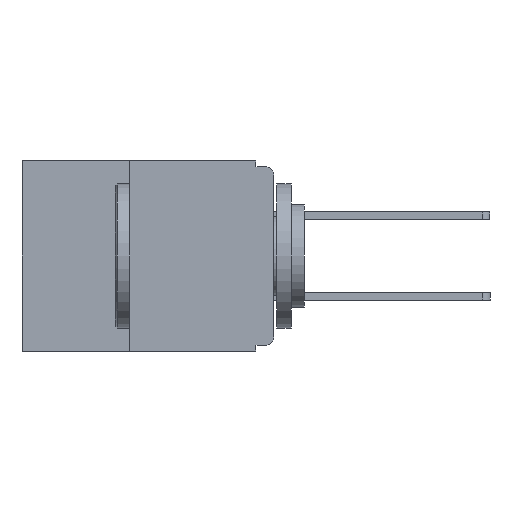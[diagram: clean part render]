
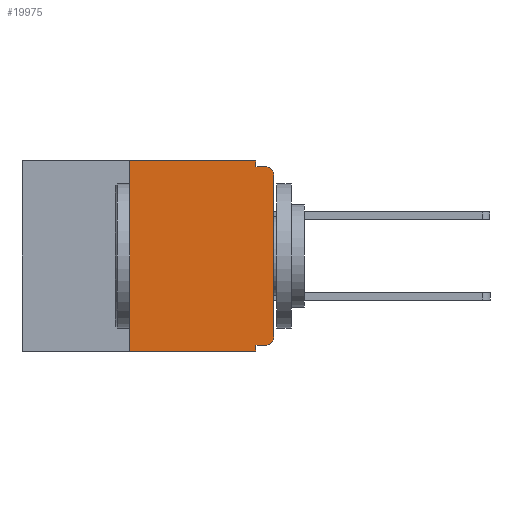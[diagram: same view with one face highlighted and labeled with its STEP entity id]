
A CAD part, left-side view. The second image highlights one B-rep face of the part: STEP entity #19975.
In plain terms, the highlighted planar face has unit normal (-1, 0, 0).
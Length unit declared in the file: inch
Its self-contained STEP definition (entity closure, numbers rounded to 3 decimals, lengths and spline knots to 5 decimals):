
#14 = DIRECTION ( 'NONE',  ( 0., 0., 1. ) ) ;
#319 = PLANE ( 'NONE',  #8817 ) ;
#542 = VERTEX_POINT ( 'NONE', #6437 ) ;
#601 = EDGE_CURVE ( 'NONE', #12210, #19480, #27100, .T. ) ;
#2142 = CARTESIAN_POINT ( 'NONE',  ( 0., 0.25, -0.33 ) ) ;
#2256 = EDGE_CURVE ( 'NONE', #4718, #12210, #6326, .T. ) ;
#2502 = LINE ( 'NONE', #9991, #25057 ) ;
#2590 = CARTESIAN_POINT ( 'NONE',  ( 0., 0.437, 0. ) ) ;
#2668 = DIRECTION ( 'NONE',  ( 0., -1., 0. ) ) ;
#2788 = CARTESIAN_POINT ( 'NONE',  ( 0., 0.25, -0.33 ) ) ;
#2958 = EDGE_LOOP ( 'NONE', ( #22342, #22671, #18648, #22723, #16633, #20723, #24435, #16682, #3962, #11297 ) ) ;
#2968 = VERTEX_POINT ( 'NONE', #4401 ) ;
#3151 = CARTESIAN_POINT ( 'NONE',  ( 0., 0., -0.32 ) ) ;
#3210 = CARTESIAN_POINT ( 'NONE',  ( 0., 0.031, -0.33 ) ) ;
#3430 = DIRECTION ( 'NONE',  ( 0., 0., -1. ) ) ;
#3502 = DIRECTION ( 'NONE',  ( 0., -1., 0. ) ) ;
#3962 = ORIENTED_EDGE ( 'NONE', *, *, #23282, .F. ) ;
#4376 = DIRECTION ( 'NONE',  ( 0., 0., 1. ) ) ;
#4401 = CARTESIAN_POINT ( 'NONE',  ( 0., 0.031, -0.32 ) ) ;
#4718 = VERTEX_POINT ( 'NONE', #13551 ) ;
#4810 = DIRECTION ( 'NONE',  ( 1., 0., 0. ) ) ;
#4890 = CARTESIAN_POINT ( 'NONE',  ( 0., 0.437, -0.33 ) ) ;
#5719 = VERTEX_POINT ( 'NONE', #17466 ) ;
#6326 = LINE ( 'NONE', #17596, #15929 ) ;
#6437 = CARTESIAN_POINT ( 'NONE',  ( 0., 0., -0.025 ) ) ;
#6845 = VECTOR ( 'NONE', #25123, 39.37008 ) ;
#7030 = DIRECTION ( 'NONE',  ( -1., 0., 0. ) ) ;
#7438 = CIRCLE ( 'NONE', #10434, 0.015 ) ;
#7445 = VECTOR ( 'NONE', #4376, 39.37008 ) ;
#8817 = AXIS2_PLACEMENT_3D ( 'NONE', #2590, #4810, #20133 ) ;
#8823 = VECTOR ( 'NONE', #2668, 39.37008 ) ;
#9991 = CARTESIAN_POINT ( 'NONE',  ( 0., 0.031, -0.33 ) ) ;
#10374 = CIRCLE ( 'NONE', #20193, 0.015 ) ;
#10434 = AXIS2_PLACEMENT_3D ( 'NONE', #11715, #26837, #13908 ) ;
#10545 = EDGE_CURVE ( 'NONE', #2968, #20801, #2502, .T. ) ;
#11297 = ORIENTED_EDGE ( 'NONE', *, *, #11732, .T. ) ;
#11715 = CARTESIAN_POINT ( 'NONE',  ( 0., 0.015, -0.025 ) ) ;
#11732 = EDGE_CURVE ( 'NONE', #14451, #21598, #10374, .T. ) ;
#12210 = VERTEX_POINT ( 'NONE', #15131 ) ;
#12665 = LINE ( 'NONE', #16422, #6845 ) ;
#13256 = LINE ( 'NONE', #2142, #7445 ) ;
#13551 = CARTESIAN_POINT ( 'NONE',  ( 0., 0.25, 0. ) ) ;
#13908 = DIRECTION ( 'NONE',  ( 0., 0., -1. ) ) ;
#14451 = VERTEX_POINT ( 'NONE', #20847 ) ;
#14544 = CARTESIAN_POINT ( 'NONE',  ( 0., 0.031, -0.01 ) ) ;
#14897 = VECTOR ( 'NONE', #14, 39.37008 ) ;
#15131 = CARTESIAN_POINT ( 'NONE',  ( 0., 0.031, 0. ) ) ;
#15929 = VECTOR ( 'NONE', #3502, 39.37008 ) ;
#16422 = CARTESIAN_POINT ( 'NONE',  ( 0., 0., -0.01 ) ) ;
#16633 = ORIENTED_EDGE ( 'NONE', *, *, #2256, .F. ) ;
#16682 = ORIENTED_EDGE ( 'NONE', *, *, #10545, .F. ) ;
#16742 = EDGE_CURVE ( 'NONE', #24988, #20801, #26151, .T. ) ;
#16828 = EDGE_CURVE ( 'NONE', #542, #5719, #7438, .T. ) ;
#17466 = CARTESIAN_POINT ( 'NONE',  ( 0., 0.015, -0.01 ) ) ;
#17543 = DIRECTION ( 'NONE',  ( 0., 0., -1. ) ) ;
#17596 = CARTESIAN_POINT ( 'NONE',  ( 0., 0.437, 0. ) ) ;
#18488 = VECTOR ( 'NONE', #18622, 39.37008 ) ;
#18622 = DIRECTION ( 'NONE',  ( 0., 1., 0. ) ) ;
#18648 = ORIENTED_EDGE ( 'NONE', *, *, #23315, .F. ) ;
#19480 = VERTEX_POINT ( 'NONE', #14544 ) ;
#19975 = ADVANCED_FACE ( 'NONE', ( #24998 ), #319, .F. ) ;
#20119 = CARTESIAN_POINT ( 'NONE',  ( 0., 0.015, -0.305 ) ) ;
#20133 = DIRECTION ( 'NONE',  ( 0., 0., -1. ) ) ;
#20193 = AXIS2_PLACEMENT_3D ( 'NONE', #20119, #7030, #22285 ) ;
#20723 = ORIENTED_EDGE ( 'NONE', *, *, #24305, .F. ) ;
#20801 = VERTEX_POINT ( 'NONE', #3210 ) ;
#20847 = CARTESIAN_POINT ( 'NONE',  ( 0., 0.015, -0.32 ) ) ;
#21598 = VERTEX_POINT ( 'NONE', #23251 ) ;
#22285 = DIRECTION ( 'NONE',  ( 0., 0., -1. ) ) ;
#22342 = ORIENTED_EDGE ( 'NONE', *, *, #25710, .T. ) ;
#22671 = ORIENTED_EDGE ( 'NONE', *, *, #16828, .T. ) ;
#22723 = ORIENTED_EDGE ( 'NONE', *, *, #601, .F. ) ;
#23251 = CARTESIAN_POINT ( 'NONE',  ( 0., 0., -0.305 ) ) ;
#23282 = EDGE_CURVE ( 'NONE', #14451, #2968, #24902, .T. ) ;
#23315 = EDGE_CURVE ( 'NONE', #19480, #5719, #12665, .T. ) ;
#24305 = EDGE_CURVE ( 'NONE', #24988, #4718, #13256, .T. ) ;
#24435 = ORIENTED_EDGE ( 'NONE', *, *, #16742, .T. ) ;
#24902 = LINE ( 'NONE', #3151, #18488 ) ;
#24988 = VERTEX_POINT ( 'NONE', #2788 ) ;
#24998 = FACE_OUTER_BOUND ( 'NONE', #2958, .T. ) ;
#25057 = VECTOR ( 'NONE', #3430, 39.37008 ) ;
#25123 = DIRECTION ( 'NONE',  ( 0., -1., 0. ) ) ;
#25353 = CARTESIAN_POINT ( 'NONE',  ( 0., 0.031, 0. ) ) ;
#25710 = EDGE_CURVE ( 'NONE', #21598, #542, #26399, .T. ) ;
#26151 = LINE ( 'NONE', #4890, #8823 ) ;
#26228 = CARTESIAN_POINT ( 'NONE',  ( 0., 0., 0. ) ) ;
#26399 = LINE ( 'NONE', #26228, #14897 ) ;
#26837 = DIRECTION ( 'NONE',  ( -1., 0., 0. ) ) ;
#27100 = LINE ( 'NONE', #25353, #27746 ) ;
#27746 = VECTOR ( 'NONE', #17543, 39.37008 ) ;
